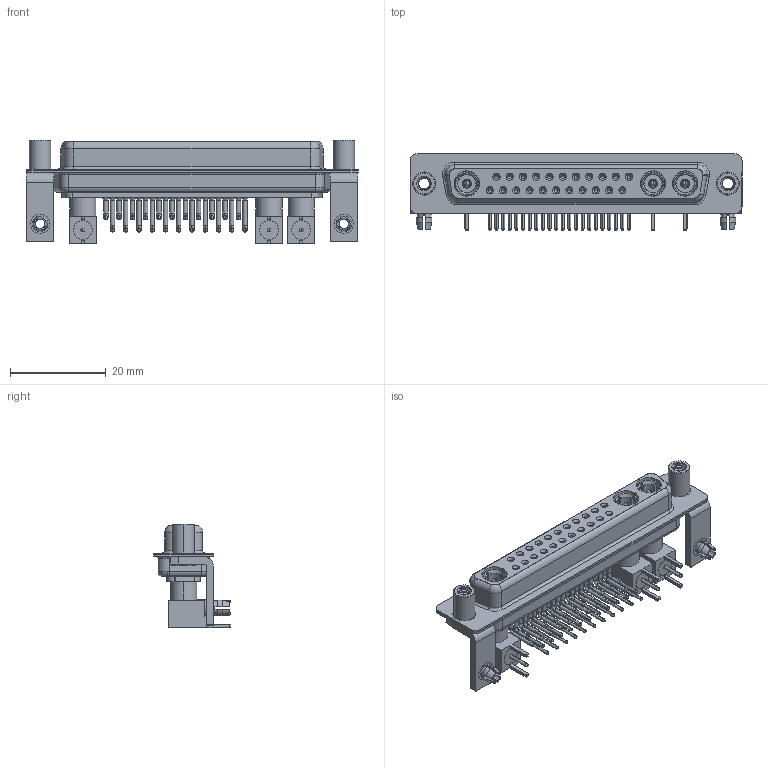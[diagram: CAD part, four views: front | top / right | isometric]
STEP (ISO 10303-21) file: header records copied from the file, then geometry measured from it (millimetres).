
FILE_DESCRIPTION (( 'STEP AP203' ), '1' );
FILE_NAME ('630-25W3240-7T5.STEP', '2022-06-07T04:18:15', ( '' ), ( '' ), 'SwSTEP 2.0', 'SolidWorks 2020', '' );
FILE_SCHEMA (( 'CONFIG_CONTROL_DESIGN' ));
Length unit declared in the file: millimetre
Products named in the file (18): Insulator Pin_Straight PC Tail; Co-Ax Plug Assy_RA; Insulator RA Pin; 630Combo Housing_25W3; RA Back Shell; 630Combo Contact Row 1; 630Combo Shell Rear_37 Contacts; 630Combo Shell Front_37 Contacts; 630-25W3240-7T5; Co-Ax Plug_RA PC Tail; Pin_RA; 630Combo Threaded Standoff_5; 630Combo Contact Row 2; 630Combo Stabilizer Bracket; Locking Collar; 630Combo Board Lock
Assembly tree (52 placements, depth 3):
  630-25W3240-7T5
    630Combo Housing_25W3
    630Combo Shell Front_37 Contacts
    630Combo Shell Rear_37 Contacts
    630Combo Stabilizer Bracket  x2
    630Combo Board Lock  x2
    630Combo Threaded Standoff_5  x2
    Co-Ax Plug Assy_RA
      Co-Ax Plug_RA PC Tail
      Insulator Pin_Straight PC Tail
      Pin_RA
      Locking Collar
      RA Back Shell
      Insulator RA Pin
    Co-Ax Plug Assy_RA
      Co-Ax Plug_RA PC Tail
      Insulator Pin_Straight PC Tail
      Pin_RA
      Locking Collar
      RA Back Shell
      Insulator RA Pin
    Co-Ax Plug Assy_RA
      Co-Ax Plug_RA PC Tail
      Insulator Pin_Straight PC Tail
      Pin_RA
      Locking Collar
      RA Back Shell
      Insulator RA Pin
    630Combo Contact Row 1  x11
    630Combo Contact Row 2  x11
Bounding box: 69.4 x 16 x 21.61 mm (x, y, z)
Volume: 6605.7 mm3; surface area: 15705.1 mm2
Topology: 49 solids, 49 shells, 2129 faces, 5342 edges, 3368 vertices
Faces by surface type: cylinder 930, plane 668, cone 347, bspline 97, torus 75, sphere 12
Entity records: 30908 total; most frequent: CARTESIAN_POINT 6865, DIRECTION 4831, ORIENTED_EDGE 4162, EDGE_CURVE 2081, AXIS2_PLACEMENT_3D 1983, VERTEX_POINT 1329, EDGE_LOOP 1058, CIRCLE 1057
